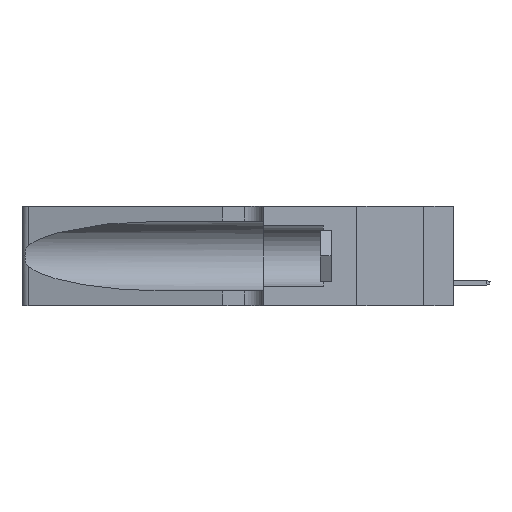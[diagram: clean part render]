
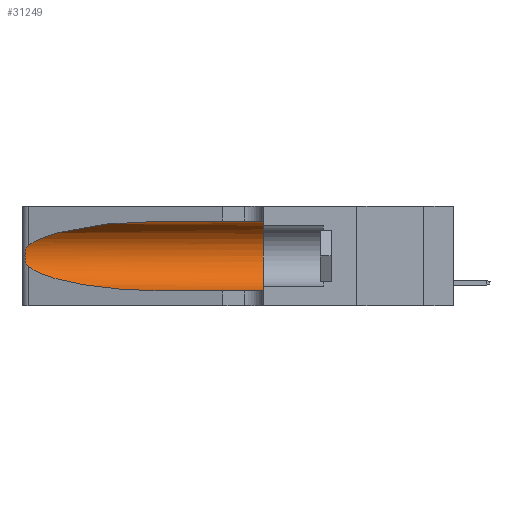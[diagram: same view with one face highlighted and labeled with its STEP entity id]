
A CAD part, left-side view. The second image highlights one B-rep face of the part: STEP entity #31249.
In plain terms, the highlighted cylindrical face has radius 3.308 mm (diameter 6.617 mm), a partial arc.
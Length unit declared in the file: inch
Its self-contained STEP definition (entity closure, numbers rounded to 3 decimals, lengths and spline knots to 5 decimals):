
#188 = CARTESIAN_POINT ( 'NONE',  ( 0.26075, 1.23896, 0.19203 ) ) ;
#991 = CARTESIAN_POINT ( 'NONE',  ( 0.1305, 0.72297, 0.31525 ) ) ;
#1793 = VERTEX_POINT ( 'NONE', #16307 ) ;
#3505 = CARTESIAN_POINT ( 'NONE',  ( 0.25787, 1.23484, 0.2124 ) ) ;
#3733 = B_SPLINE_CURVE_WITH_KNOTS ( 'NONE', 3,
 ( #20596, #20808, #14154, #3505, #7074, #27463, #188, #24339, #27688, #10819, #16820, #20152, #20368, #31250 ),
 .UNSPECIFIED., .F., .F.,
 ( 4, 2, 2, 2, 2, 2, 4 ),
 ( 0., 0.00027, 0.00053, 0.00107, 0.0016, 0.00187, 0.00214 ),
 .UNSPECIFIED. ) ;
#3748 = ORIENTED_EDGE ( 'NONE', *, *, #12822, .F. ) ;
#3957 = CARTESIAN_POINT ( 'NONE',  ( 0.1305, 0.35, 0.05475 ) ) ;
#4514 = VERTEX_POINT ( 'NONE', #3957 ) ;
#4942 = LINE ( 'NONE', #22246, #6916 ) ;
#6583 = VERTEX_POINT ( 'NONE', #20943 ) ;
#6832 = DIRECTION ( 'NONE',  ( 0., -1., 0. ) ) ;
#6916 = VECTOR ( 'NONE', #32240, 39.37008 ) ;
#6919 = CARTESIAN_POINT ( 'NONE',  ( 0.2373, 1.15595, 0.28018 ) ) ;
#7074 = CARTESIAN_POINT ( 'NONE',  ( 0.25854, 1.2359, 0.20912 ) ) ;
#8336 = DIRECTION ( 'NONE',  ( 0., -1., 0. ) ) ;
#8896 = EDGE_CURVE ( 'NONE', #31575, #4514, #9175, .T. ) ;
#9175 = LINE ( 'NONE', #36468, #42410 ) ;
#10249 = ORIENTED_EDGE ( 'NONE', *, *, #8896, .T. ) ;
#10357 = CARTESIAN_POINT ( 'NONE',  ( 0.1305, 1.61858, 0.185 ) ) ;
#10819 = CARTESIAN_POINT ( 'NONE',  ( 0.25856, 1.23593, 0.16098 ) ) ;
#11177 = CARTESIAN_POINT ( 'NONE',  ( 0.1305, 0.72297, 0.05475 ) ) ;
#11637 = ORIENTED_EDGE ( 'NONE', *, *, #17293, .T. ) ;
#11747 = VERTEX_POINT ( 'NONE', #34088 ) ;
#12822 = EDGE_CURVE ( 'NONE', #1793, #4514, #37601, .T. ) ;
#13547 = CARTESIAN_POINT ( 'NONE',  ( 0.18966, 0.96281, 0.05475 ) ) ;
#14154 = CARTESIAN_POINT ( 'NONE',  ( 0.25639, 1.23184, 0.21858 ) ) ;
#16139 = EDGE_LOOP ( 'NONE', ( #11637, #16639, #41271, #10249, #3748, #40802 ) ) ;
#16307 = CARTESIAN_POINT ( 'NONE',  ( 0.1305, 0.35, 0.31525 ) ) ;
#16639 = ORIENTED_EDGE ( 'NONE', *, *, #24603, .T. ) ;
#16820 = CARTESIAN_POINT ( 'NONE',  ( 0.25789, 1.23486, 0.15765 ) ) ;
#17020 = FACE_OUTER_BOUND ( 'NONE', #16139, .T. ) ;
#17293 = EDGE_CURVE ( 'NONE', #34255, #11747, #26170, .T. ) ;
#18188 = DIRECTION ( 'NONE',  ( 0., 0., 1. ) ) ;
#20152 = CARTESIAN_POINT ( 'NONE',  ( 0.25639, 1.23186, 0.15144 ) ) ;
#20368 = CARTESIAN_POINT ( 'NONE',  ( 0.25555, 1.22993, 0.14849 ) ) ;
#20411 = CARTESIAN_POINT ( 'NONE',  ( 0.2373, 1.15595, 0.08982 ) ) ;
#20596 = CARTESIAN_POINT ( 'NONE',  ( 0.25487, 1.22718, 0.22369 ) ) ;
#20662 = CARTESIAN_POINT ( 'NONE',  ( 0.18966, 0.96281, 0.31525 ) ) ;
#20808 = CARTESIAN_POINT ( 'NONE',  ( 0.25555, 1.22994, 0.2215 ) ) ;
#20943 = CARTESIAN_POINT ( 'NONE',  ( 0.25487, 1.22718, 0.14631 ) ) ;
#21278 = AXIS2_PLACEMENT_3D ( 'NONE', #41977, #21535, #18188 ) ;
#21535 = DIRECTION ( 'NONE',  ( 0., 1., 0. ) ) ;
#21574 = EDGE_CURVE ( 'NONE', #34255, #1793, #4942, .T. ) ;
#22246 = CARTESIAN_POINT ( 'NONE',  ( 0.1305, 1.61858, 0.31525 ) ) ;
#24339 = CARTESIAN_POINT ( 'NONE',  ( 0.26075, 1.23896, 0.178 ) ) ;
#24535 = CYLINDRICAL_SURFACE ( 'NONE', #32286, 0.13025 ) ;
#24603 = EDGE_CURVE ( 'NONE', #11747, #6583, #3733, .T. ) ;
#26170 =( BOUNDED_CURVE ( )  B_SPLINE_CURVE ( 3, ( #34194, #20662, #6919, #27313 ),
 .UNSPECIFIED., .F., .T. ) 
 B_SPLINE_CURVE_WITH_KNOTS ( ( 4, 4 ),
 ( 1.5708, 2.84003 ),
 .UNSPECIFIED. ) 
 CURVE ( )  GEOMETRIC_REPRESENTATION_ITEM ( )  RATIONAL_B_SPLINE_CURVE ( ( 1., 0.87, 0.87, 1. ) ) 
 REPRESENTATION_ITEM ( '' )  );
#27313 = CARTESIAN_POINT ( 'NONE',  ( 0.25487, 1.22718, 0.22369 ) ) ;
#27463 = CARTESIAN_POINT ( 'NONE',  ( 0.26018, 1.23835, 0.19895 ) ) ;
#27688 = CARTESIAN_POINT ( 'NONE',  ( 0.26017, 1.23833, 0.17102 ) ) ;
#27836 = EDGE_CURVE ( 'NONE', #6583, #31575, #41735, .T. ) ;
#31249 = ADVANCED_FACE ( 'NONE', ( #17020 ), #24535, .F. ) ;
#31250 = CARTESIAN_POINT ( 'NONE',  ( 0.25487, 1.22718, 0.14631 ) ) ;
#31575 = VERTEX_POINT ( 'NONE', #11177 ) ;
#32240 = DIRECTION ( 'NONE',  ( 0., -1., 0. ) ) ;
#32286 = AXIS2_PLACEMENT_3D ( 'NONE', #10357, #6832, #33893 ) ;
#33893 = DIRECTION ( 'NONE',  ( 0., 0., -1. ) ) ;
#33957 = CARTESIAN_POINT ( 'NONE',  ( 0.1305, 0.72297, 0.05475 ) ) ;
#34088 = CARTESIAN_POINT ( 'NONE',  ( 0.25487, 1.22718, 0.22369 ) ) ;
#34194 = CARTESIAN_POINT ( 'NONE',  ( 0.1305, 0.72297, 0.31525 ) ) ;
#34255 = VERTEX_POINT ( 'NONE', #991 ) ;
#36468 = CARTESIAN_POINT ( 'NONE',  ( 0.1305, 1.61858, 0.05475 ) ) ;
#37601 = CIRCLE ( 'NONE', #21278, 0.13025 ) ;
#39777 = CARTESIAN_POINT ( 'NONE',  ( 0.25487, 1.22718, 0.14631 ) ) ;
#40802 = ORIENTED_EDGE ( 'NONE', *, *, #21574, .F. ) ;
#41271 = ORIENTED_EDGE ( 'NONE', *, *, #27836, .T. ) ;
#41735 =( BOUNDED_CURVE ( )  B_SPLINE_CURVE ( 3, ( #39777, #20411, #13547, #33957 ),
 .UNSPECIFIED., .F., .T. ) 
 B_SPLINE_CURVE_WITH_KNOTS ( ( 4, 4 ),
 ( 3.44316, 4.71239 ),
 .UNSPECIFIED. ) 
 CURVE ( )  GEOMETRIC_REPRESENTATION_ITEM ( )  RATIONAL_B_SPLINE_CURVE ( ( 1., 0.87, 0.87, 1. ) ) 
 REPRESENTATION_ITEM ( '' )  );
#41977 = CARTESIAN_POINT ( 'NONE',  ( 0.1305, 0.35, 0.185 ) ) ;
#42410 = VECTOR ( 'NONE', #8336, 39.37008 ) ;
